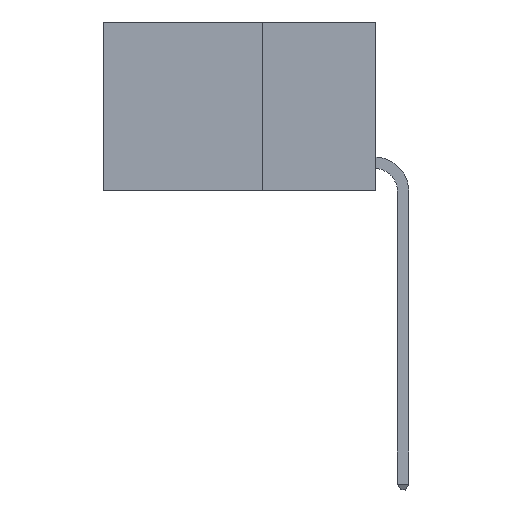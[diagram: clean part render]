
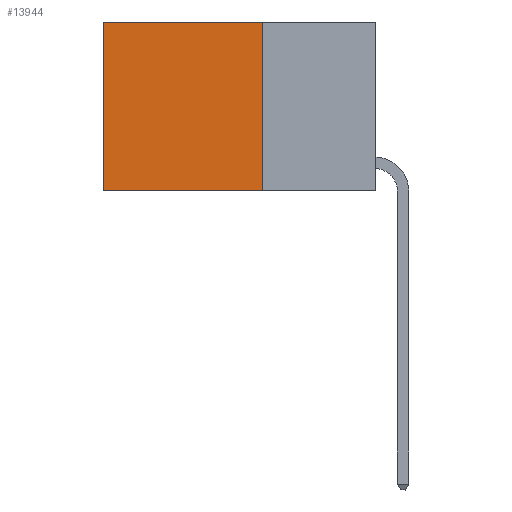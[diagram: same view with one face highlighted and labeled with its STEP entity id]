
A CAD part, left-side view. The second image highlights one B-rep face of the part: STEP entity #13944.
In plain terms, the highlighted planar face has unit normal (-1, 0, 0).
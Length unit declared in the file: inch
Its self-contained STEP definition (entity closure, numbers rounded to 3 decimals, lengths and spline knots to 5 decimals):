
#61 = DIRECTION ( 'NONE',  ( 0., 0., -1. ) ) ;
#119 = VECTOR ( 'NONE', #8630, 39.37008 ) ;
#902 = VERTEX_POINT ( 'NONE', #966 ) ;
#966 = CARTESIAN_POINT ( 'NONE',  ( 0.2625, 0.25, -0.37 ) ) ;
#1594 = ORIENTED_EDGE ( 'NONE', *, *, #5341, .F. ) ;
#1630 = VERTEX_POINT ( 'NONE', #10561 ) ;
#2437 = CARTESIAN_POINT ( 'NONE',  ( 0.2625, 0.6, 0. ) ) ;
#2845 = EDGE_CURVE ( 'NONE', #13902, #14324, #13202, .T. ) ;
#3211 = CARTESIAN_POINT ( 'NONE',  ( 0.2625, 0.25, 0. ) ) ;
#4149 = EDGE_LOOP ( 'NONE', ( #9414, #1594, #13295, #13050 ) ) ;
#5341 = EDGE_CURVE ( 'NONE', #902, #14324, #14499, .T. ) ;
#6015 = PLANE ( 'NONE',  #9405 ) ;
#7144 = DIRECTION ( 'NONE',  ( 1., 0., 0. ) ) ;
#8089 = LINE ( 'NONE', #13982, #10701 ) ;
#8141 = CARTESIAN_POINT ( 'NONE',  ( 0.2625, 0.6, 0. ) ) ;
#8187 = DIRECTION ( 'NONE',  ( 0., 0., -1. ) ) ;
#8531 = DIRECTION ( 'NONE',  ( 0., 0., -1. ) ) ;
#8630 = DIRECTION ( 'NONE',  ( 0., 1., 0. ) ) ;
#8890 = EDGE_CURVE ( 'NONE', #1630, #902, #8089, .T. ) ;
#9405 = AXIS2_PLACEMENT_3D ( 'NONE', #13700, #7144, #61 ) ;
#9414 = ORIENTED_EDGE ( 'NONE', *, *, #2845, .T. ) ;
#10012 = DIRECTION ( 'NONE',  ( 0., 1., 0. ) ) ;
#10015 = CARTESIAN_POINT ( 'NONE',  ( 0.2625, 0.6, -0.37 ) ) ;
#10561 = CARTESIAN_POINT ( 'NONE',  ( 0.2625, 0.25, 0. ) ) ;
#10701 = VECTOR ( 'NONE', #8531, 39.37008 ) ;
#11235 = FACE_OUTER_BOUND ( 'NONE', #4149, .T. ) ;
#11660 = EDGE_CURVE ( 'NONE', #1630, #13902, #14657, .T. ) ;
#12871 = VECTOR ( 'NONE', #8187, 39.37008 ) ;
#13050 = ORIENTED_EDGE ( 'NONE', *, *, #11660, .T. ) ;
#13202 = LINE ( 'NONE', #2437, #12871 ) ;
#13295 = ORIENTED_EDGE ( 'NONE', *, *, #8890, .F. ) ;
#13700 = CARTESIAN_POINT ( 'NONE',  ( 0.2625, 0.25, 0. ) ) ;
#13902 = VERTEX_POINT ( 'NONE', #8141 ) ;
#13944 = ADVANCED_FACE ( 'NONE', ( #11235 ), #6015, .F. ) ;
#13982 = CARTESIAN_POINT ( 'NONE',  ( 0.2625, 0.25, 0. ) ) ;
#14075 = CARTESIAN_POINT ( 'NONE',  ( 0.2625, 0.25, -0.37 ) ) ;
#14300 = VECTOR ( 'NONE', #10012, 39.37008 ) ;
#14324 = VERTEX_POINT ( 'NONE', #10015 ) ;
#14499 = LINE ( 'NONE', #14075, #119 ) ;
#14657 = LINE ( 'NONE', #3211, #14300 ) ;
